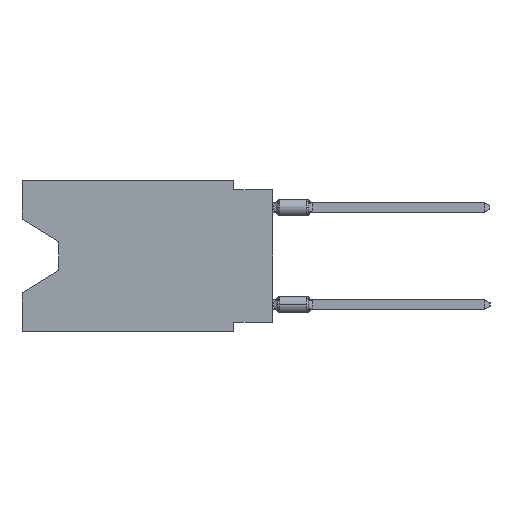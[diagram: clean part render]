
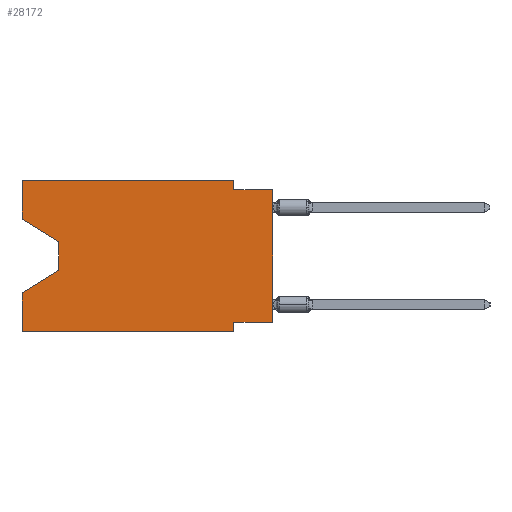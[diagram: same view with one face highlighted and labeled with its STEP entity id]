
A CAD part, left-side view. The second image highlights one B-rep face of the part: STEP entity #28172.
In plain terms, the highlighted planar face has unit normal (-1, 0, 0).
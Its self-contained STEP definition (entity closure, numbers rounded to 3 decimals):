
#591 = LINE ( 'NONE', #22824, #46560 ) ;
#744 = VECTOR ( 'NONE', #63537, 1000. ) ;
#2409 = CARTESIAN_POINT ( 'NONE',  ( 0., 16.383, -9.906 ) ) ;
#2691 = VERTEX_POINT ( 'NONE', #23216 ) ;
#3215 = ORIENTED_EDGE ( 'NONE', *, *, #10864, .F. ) ;
#5209 = ORIENTED_EDGE ( 'NONE', *, *, #21316, .T. ) ;
#5744 = CARTESIAN_POINT ( 'NONE',  ( 0., 0., -9.271 ) ) ;
#5812 = ORIENTED_EDGE ( 'NONE', *, *, #17144, .F. ) ;
#7011 = DIRECTION ( 'NONE',  ( 0., 1., 0. ) ) ;
#9966 = LINE ( 'NONE', #50001, #44837 ) ;
#10864 = EDGE_CURVE ( 'NONE', #24247, #55490, #48954, .T. ) ;
#12013 = VERTEX_POINT ( 'NONE', #29640 ) ;
#12041 = ORIENTED_EDGE ( 'NONE', *, *, #35100, .T. ) ;
#12281 = CARTESIAN_POINT ( 'NONE',  ( 0., 16.383, -2.546 ) ) ;
#12749 = CARTESIAN_POINT ( 'NONE',  ( 0., 13.97, -5.893 ) ) ;
#13109 = DIRECTION ( 'NONE',  ( 0., -1., 0. ) ) ;
#14017 = ORIENTED_EDGE ( 'NONE', *, *, #42800, .F. ) ;
#14609 = CARTESIAN_POINT ( 'NONE',  ( 0., 0., -0.635 ) ) ;
#14700 = CARTESIAN_POINT ( 'NONE',  ( 0., 13.97, -5.893 ) ) ;
#16562 = VERTEX_POINT ( 'NONE', #63211 ) ;
#16707 = FACE_OUTER_BOUND ( 'NONE', #60489, .T. ) ;
#16760 = EDGE_CURVE ( 'NONE', #38037, #2691, #37249, .T. ) ;
#17144 = EDGE_CURVE ( 'NONE', #12013, #52820, #9966, .T. ) ;
#18830 = EDGE_CURVE ( 'NONE', #55490, #21662, #23994, .T. ) ;
#18979 = CARTESIAN_POINT ( 'NONE',  ( 0., 0., -0.635 ) ) ;
#21316 = EDGE_CURVE ( 'NONE', #12013, #16562, #47339, .T. ) ;
#21662 = VERTEX_POINT ( 'NONE', #61395 ) ;
#21987 = VECTOR ( 'NONE', #26075, 1000. ) ;
#22824 = CARTESIAN_POINT ( 'NONE',  ( 0., 16.383, 0. ) ) ;
#23216 = CARTESIAN_POINT ( 'NONE',  ( 0., 13.97, -4.013 ) ) ;
#23994 = LINE ( 'NONE', #36774, #41833 ) ;
#24247 = VERTEX_POINT ( 'NONE', #52082 ) ;
#24446 = EDGE_CURVE ( 'NONE', #2691, #33709, #25441, .T. ) ;
#24552 = LINE ( 'NONE', #14700, #64616 ) ;
#25251 = CARTESIAN_POINT ( 'NONE',  ( 0., 16.383, -7.36 ) ) ;
#25441 = LINE ( 'NONE', #54661, #21987 ) ;
#26075 = DIRECTION ( 'NONE',  ( 0., 0., -1. ) ) ;
#28172 = ADVANCED_FACE ( 'NONE', ( #16707 ), #50860, .F. ) ;
#28734 = ORIENTED_EDGE ( 'NONE', *, *, #35455, .F. ) ;
#29640 = CARTESIAN_POINT ( 'NONE',  ( 0., 16.383, -9.906 ) ) ;
#29813 = DIRECTION ( 'NONE',  ( 0., 0.855, -0.519 ) ) ;
#30923 = ORIENTED_EDGE ( 'NONE', *, *, #24446, .T. ) ;
#31631 = CARTESIAN_POINT ( 'NONE',  ( 0., 0., -9.271 ) ) ;
#31900 = VECTOR ( 'NONE', #57510, 1000. ) ;
#32685 = EDGE_CURVE ( 'NONE', #40732, #57232, #45436, .T. ) ;
#32987 = VECTOR ( 'NONE', #13109, 1000. ) ;
#33709 = VERTEX_POINT ( 'NONE', #12749 ) ;
#34552 = VECTOR ( 'NONE', #58800, 1000. ) ;
#35100 = EDGE_CURVE ( 'NONE', #33709, #52820, #24552, .T. ) ;
#35396 = EDGE_CURVE ( 'NONE', #40732, #41617, #42875, .T. ) ;
#35455 = EDGE_CURVE ( 'NONE', #57232, #16562, #38298, .T. ) ;
#36106 = DIRECTION ( 'NONE',  ( 0., 0., -1. ) ) ;
#36774 = CARTESIAN_POINT ( 'NONE',  ( 0., 2.54, 0. ) ) ;
#37249 = LINE ( 'NONE', #12281, #52101 ) ;
#37965 = DIRECTION ( 'NONE',  ( 0., 0., 1. ) ) ;
#38037 = VERTEX_POINT ( 'NONE', #48199 ) ;
#38298 = LINE ( 'NONE', #54657, #744 ) ;
#39443 = CARTESIAN_POINT ( 'NONE',  ( 0., 16.383, 0. ) ) ;
#40732 = VERTEX_POINT ( 'NONE', #31631 ) ;
#41617 = VERTEX_POINT ( 'NONE', #14609 ) ;
#41693 = DIRECTION ( 'NONE',  ( 0., 0., -1. ) ) ;
#41833 = VECTOR ( 'NONE', #41693, 1000. ) ;
#42800 = EDGE_CURVE ( 'NONE', #21662, #41617, #47894, .T. ) ;
#42875 = LINE ( 'NONE', #48118, #50970 ) ;
#43355 = CARTESIAN_POINT ( 'NONE',  ( 0., 2.54, 0. ) ) ;
#43665 = ORIENTED_EDGE ( 'NONE', *, *, #18830, .F. ) ;
#44837 = VECTOR ( 'NONE', #45061, 1000. ) ;
#45061 = DIRECTION ( 'NONE',  ( 0., 0., 1. ) ) ;
#45436 = LINE ( 'NONE', #5744, #59142 ) ;
#46560 = VECTOR ( 'NONE', #56320, 1000. ) ;
#46756 = DIRECTION ( 'NONE',  ( 0., -0.855, -0.519 ) ) ;
#47339 = LINE ( 'NONE', #2409, #31900 ) ;
#47457 = AXIS2_PLACEMENT_3D ( 'NONE', #61017, #55453, #36106 ) ;
#47894 = LINE ( 'NONE', #18979, #32987 ) ;
#48118 = CARTESIAN_POINT ( 'NONE',  ( 0., 0., 0. ) ) ;
#48199 = CARTESIAN_POINT ( 'NONE',  ( 0., 16.383, -2.546 ) ) ;
#48954 = LINE ( 'NONE', #39443, #34552 ) ;
#50001 = CARTESIAN_POINT ( 'NONE',  ( 0., 16.383, 0. ) ) ;
#50860 = PLANE ( 'NONE',  #47457 ) ;
#50970 = VECTOR ( 'NONE', #37965, 1000. ) ;
#52082 = CARTESIAN_POINT ( 'NONE',  ( 0., 16.383, 0. ) ) ;
#52101 = VECTOR ( 'NONE', #46756, 1000. ) ;
#52820 = VERTEX_POINT ( 'NONE', #25251 ) ;
#54657 = CARTESIAN_POINT ( 'NONE',  ( 0., 2.54, -9.906 ) ) ;
#54661 = CARTESIAN_POINT ( 'NONE',  ( 0., 13.97, -4.013 ) ) ;
#55453 = DIRECTION ( 'NONE',  ( 1., 0., 0. ) ) ;
#55490 = VERTEX_POINT ( 'NONE', #43355 ) ;
#56320 = DIRECTION ( 'NONE',  ( 0., 0., 1. ) ) ;
#56547 = ORIENTED_EDGE ( 'NONE', *, *, #32685, .F. ) ;
#57232 = VERTEX_POINT ( 'NONE', #60628 ) ;
#57470 = ORIENTED_EDGE ( 'NONE', *, *, #16760, .T. ) ;
#57510 = DIRECTION ( 'NONE',  ( 0., -1., 0. ) ) ;
#58800 = DIRECTION ( 'NONE',  ( 0., -1., 0. ) ) ;
#59142 = VECTOR ( 'NONE', #7011, 1000. ) ;
#60489 = EDGE_LOOP ( 'NONE', ( #57470, #30923, #12041, #5812, #5209, #28734, #56547, #60549, #14017, #43665, #3215, #63466 ) ) ;
#60549 = ORIENTED_EDGE ( 'NONE', *, *, #35396, .T. ) ;
#60628 = CARTESIAN_POINT ( 'NONE',  ( 0., 2.54, -9.271 ) ) ;
#61017 = CARTESIAN_POINT ( 'NONE',  ( 0., 16.383, 0. ) ) ;
#61395 = CARTESIAN_POINT ( 'NONE',  ( 0., 2.54, -0.635 ) ) ;
#63211 = CARTESIAN_POINT ( 'NONE',  ( 0., 2.54, -9.906 ) ) ;
#63466 = ORIENTED_EDGE ( 'NONE', *, *, #63685, .F. ) ;
#63537 = DIRECTION ( 'NONE',  ( 0., 0., -1. ) ) ;
#63685 = EDGE_CURVE ( 'NONE', #38037, #24247, #591, .T. ) ;
#64616 = VECTOR ( 'NONE', #29813, 1000. ) ;
